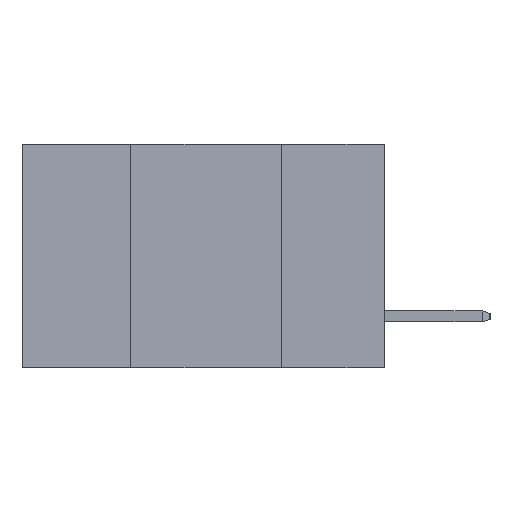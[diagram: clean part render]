
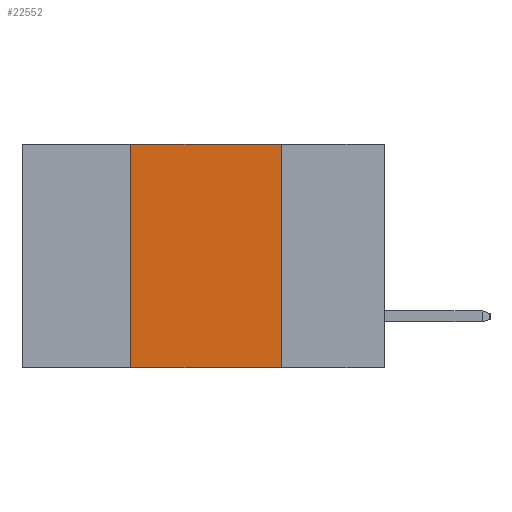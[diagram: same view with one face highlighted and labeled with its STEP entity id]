
A CAD part, left-side view. The second image highlights one B-rep face of the part: STEP entity #22552.
In plain terms, the highlighted planar face has unit normal (-1, 0, 0).
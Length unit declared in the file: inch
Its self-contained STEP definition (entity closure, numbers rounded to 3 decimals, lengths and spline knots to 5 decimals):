
#1271 = EDGE_CURVE ( 'NONE', #5745, #14641, #25270, .T. ) ;
#1512 = DIRECTION ( 'NONE',  ( 0., 0., 1. ) ) ;
#3880 = FACE_OUTER_BOUND ( 'NONE', #28487, .T. ) ;
#4424 = LINE ( 'NONE', #14110, #21708 ) ;
#4488 = CARTESIAN_POINT ( 'NONE',  ( 0., 0.6, 0. ) ) ;
#5745 = VERTEX_POINT ( 'NONE', #20873 ) ;
#7595 = PLANE ( 'NONE',  #19276 ) ;
#8421 = VECTOR ( 'NONE', #16228, 39.37008 ) ;
#8473 = VERTEX_POINT ( 'NONE', #11945 ) ;
#9907 = DIRECTION ( 'NONE',  ( 0., 0., -1. ) ) ;
#11945 = CARTESIAN_POINT ( 'NONE',  ( 0., 0.17, 0. ) ) ;
#12061 = EDGE_CURVE ( 'NONE', #5745, #13676, #13025, .T. ) ;
#12366 = EDGE_CURVE ( 'NONE', #8473, #13676, #4424, .T. ) ;
#13025 = LINE ( 'NONE', #17008, #8421 ) ;
#13440 = CARTESIAN_POINT ( 'NONE',  ( 0., 0.17, -0.37 ) ) ;
#13676 = VERTEX_POINT ( 'NONE', #13440 ) ;
#13851 = DIRECTION ( 'NONE',  ( 0., 0., -1. ) ) ;
#13918 = LINE ( 'NONE', #4488, #19173 ) ;
#14110 = CARTESIAN_POINT ( 'NONE',  ( 0., 0.17, 0. ) ) ;
#14641 = VERTEX_POINT ( 'NONE', #21469 ) ;
#14958 = EDGE_CURVE ( 'NONE', #14641, #8473, #13918, .T. ) ;
#16228 = DIRECTION ( 'NONE',  ( 0., -1., 0. ) ) ;
#17008 = CARTESIAN_POINT ( 'NONE',  ( 0., 0.6, -0.37 ) ) ;
#18180 = ORIENTED_EDGE ( 'NONE', *, *, #1271, .F. ) ;
#18794 = CARTESIAN_POINT ( 'NONE',  ( 0., 0.6, 0. ) ) ;
#19173 = VECTOR ( 'NONE', #28888, 39.37008 ) ;
#19276 = AXIS2_PLACEMENT_3D ( 'NONE', #18794, #23253, #9907 ) ;
#20040 = ORIENTED_EDGE ( 'NONE', *, *, #14958, .F. ) ;
#20873 = CARTESIAN_POINT ( 'NONE',  ( 0., 0.42, -0.37 ) ) ;
#21177 = ORIENTED_EDGE ( 'NONE', *, *, #12061, .T. ) ;
#21469 = CARTESIAN_POINT ( 'NONE',  ( 0., 0.42, 0. ) ) ;
#21708 = VECTOR ( 'NONE', #13851, 39.37008 ) ;
#22552 = ADVANCED_FACE ( 'NONE', ( #3880 ), #7595, .F. ) ;
#23253 = DIRECTION ( 'NONE',  ( 1., 0., 0. ) ) ;
#23257 = VECTOR ( 'NONE', #1512, 39.37008 ) ;
#25270 = LINE ( 'NONE', #26168, #23257 ) ;
#26168 = CARTESIAN_POINT ( 'NONE',  ( 0., 0.42, 0. ) ) ;
#28487 = EDGE_LOOP ( 'NONE', ( #28528, #20040, #18180, #21177 ) ) ;
#28528 = ORIENTED_EDGE ( 'NONE', *, *, #12366, .F. ) ;
#28888 = DIRECTION ( 'NONE',  ( 0., -1., 0. ) ) ;
